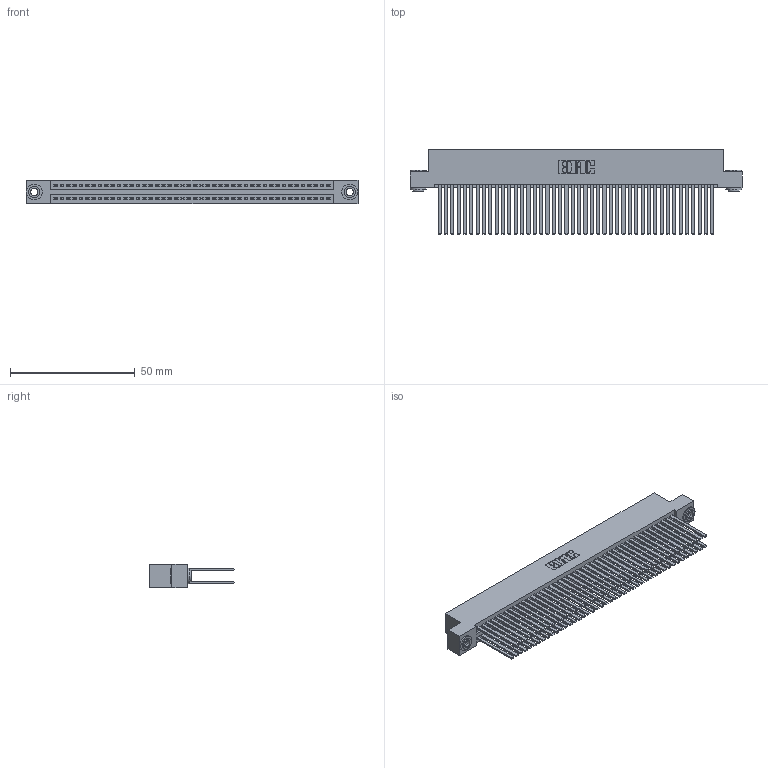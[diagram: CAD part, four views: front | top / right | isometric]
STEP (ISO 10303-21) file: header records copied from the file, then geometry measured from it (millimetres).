
FILE_DESCRIPTION (( 'STEP AP203' ), '1' );
FILE_NAME ('345-088-544-203.STEP', '2019-11-01T13:03:41', ( '' ), ( '' ), 'SwSTEP 2.0', 'SolidWorks 2016', '' );
FILE_SCHEMA (( 'CONFIG_CONTROL_DESIGN' ));
Length unit declared in the file: inch
Products named in the file (4): 345-088-544-203; 345 Part_Flush Mounting Lugs - 0.156 Dia-TH; 345-292-001_345-293-144; 345-250-002_345-250-002-102
Assembly tree (91 placements, depth 2):
  345-088-544-203
    345 Part_Flush Mounting Lugs - 0.156 Dia-TH
    345-292-001_345-293-144  x88
    345-250-002_345-250-002-102  x2
Bounding box: 132.97 x 33.96 x 9.4 mm (x, y, z)
Volume: 14188.3 mm3; surface area: 24831.9 mm2
Topology: 91 solids, 91 shells, 4036 faces, 11945 edges, 7842 vertices
Faces by surface type: plane 2642, cylinder 1386, cone 8
Entity records: 34720 total; most frequent: CARTESIAN_POINT 5791, ORIENTED_EDGE 5718, DIRECTION 5133, EDGE_CURVE 2859, VECTOR 2531, LINE 2531, VERTEX_POINT 1902, AXIS2_PLACEMENT_3D 1301
